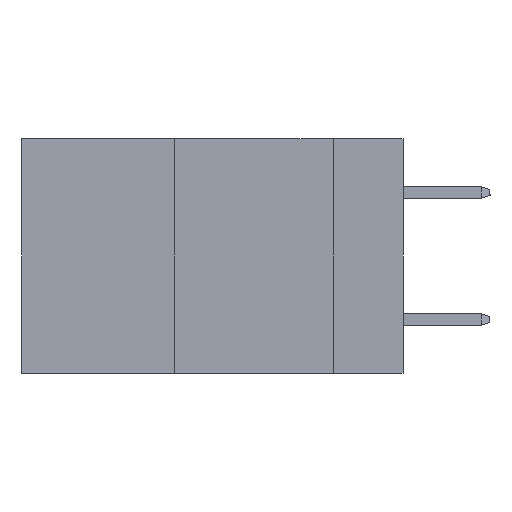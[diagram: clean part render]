
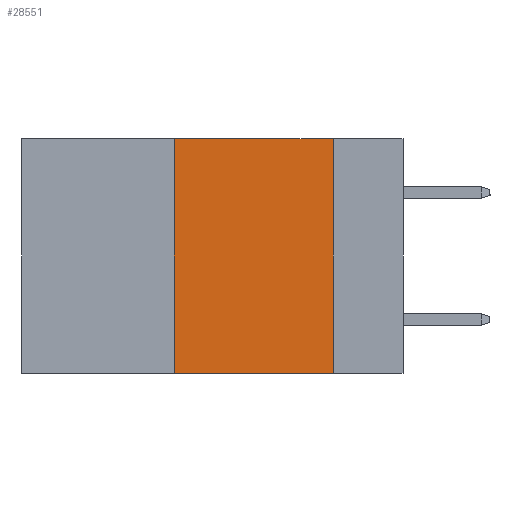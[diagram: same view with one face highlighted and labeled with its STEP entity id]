
A CAD part, left-side view. The second image highlights one B-rep face of the part: STEP entity #28551.
In plain terms, the highlighted planar face has unit normal (-1, 0, 0).
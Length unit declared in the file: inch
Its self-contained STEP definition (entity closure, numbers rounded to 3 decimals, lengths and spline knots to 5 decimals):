
#2317 = LINE ( 'NONE', #31245, #19670 ) ;
#3400 = ORIENTED_EDGE ( 'NONE', *, *, #35143, .F. ) ;
#4160 = LINE ( 'NONE', #34014, #9549 ) ;
#4209 = EDGE_CURVE ( 'NONE', #11632, #8335, #40789, .T. ) ;
#4384 = EDGE_LOOP ( 'NONE', ( #42977, #7001, #3400, #21047 ) ) ;
#6103 = VERTEX_POINT ( 'NONE', #44693 ) ;
#7001 = ORIENTED_EDGE ( 'NONE', *, *, #28301, .F. ) ;
#7663 = CARTESIAN_POINT ( 'NONE',  ( 0., 0.11, 0. ) ) ;
#7670 = CARTESIAN_POINT ( 'NONE',  ( 0., 0.36, -0.37 ) ) ;
#8335 = VERTEX_POINT ( 'NONE', #31499 ) ;
#9549 = VECTOR ( 'NONE', #26662, 39.37008 ) ;
#11632 = VERTEX_POINT ( 'NONE', #7670 ) ;
#12111 = DIRECTION ( 'NONE',  ( 0., 0., -1. ) ) ;
#13612 = EDGE_CURVE ( 'NONE', #15372, #8335, #19230, .T. ) ;
#15196 = CARTESIAN_POINT ( 'NONE',  ( 0., 0.11, 0. ) ) ;
#15372 = VERTEX_POINT ( 'NONE', #7663 ) ;
#19230 = LINE ( 'NONE', #15196, #39089 ) ;
#19670 = VECTOR ( 'NONE', #45721, 39.37008 ) ;
#21047 = ORIENTED_EDGE ( 'NONE', *, *, #4209, .T. ) ;
#26662 = DIRECTION ( 'NONE',  ( 0., -1., 0. ) ) ;
#27371 = PLANE ( 'NONE',  #33815 ) ;
#28301 = EDGE_CURVE ( 'NONE', #6103, #15372, #4160, .T. ) ;
#28551 = ADVANCED_FACE ( 'NONE', ( #45392 ), #27371, .F. ) ;
#28554 = DIRECTION ( 'NONE',  ( 0., 0., -1. ) ) ;
#28994 = VECTOR ( 'NONE', #33921, 39.37008 ) ;
#31245 = CARTESIAN_POINT ( 'NONE',  ( 0., 0.36, 0. ) ) ;
#31499 = CARTESIAN_POINT ( 'NONE',  ( 0., 0.11, -0.37 ) ) ;
#33815 = AXIS2_PLACEMENT_3D ( 'NONE', #41828, #43233, #28554 ) ;
#33921 = DIRECTION ( 'NONE',  ( 0., -1., 0. ) ) ;
#34014 = CARTESIAN_POINT ( 'NONE',  ( 0., 0.6, 0. ) ) ;
#35143 = EDGE_CURVE ( 'NONE', #11632, #6103, #2317, .T. ) ;
#37710 = CARTESIAN_POINT ( 'NONE',  ( 0., 0.6, -0.37 ) ) ;
#39089 = VECTOR ( 'NONE', #12111, 39.37008 ) ;
#40789 = LINE ( 'NONE', #37710, #28994 ) ;
#41828 = CARTESIAN_POINT ( 'NONE',  ( 0., 0.6, 0. ) ) ;
#42977 = ORIENTED_EDGE ( 'NONE', *, *, #13612, .F. ) ;
#43233 = DIRECTION ( 'NONE',  ( 1., 0., 0. ) ) ;
#44693 = CARTESIAN_POINT ( 'NONE',  ( 0., 0.36, 0. ) ) ;
#45392 = FACE_OUTER_BOUND ( 'NONE', #4384, .T. ) ;
#45721 = DIRECTION ( 'NONE',  ( 0., 0., 1. ) ) ;
